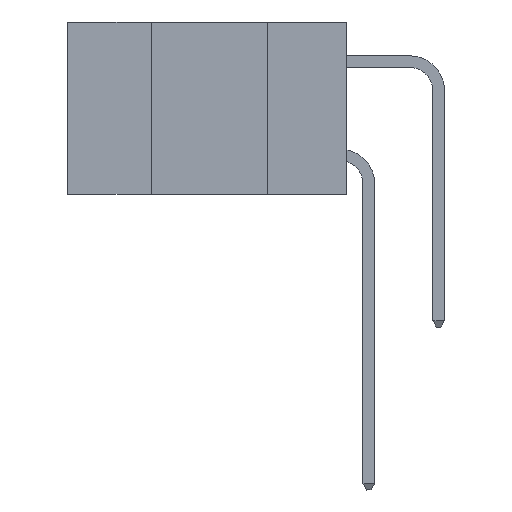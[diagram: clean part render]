
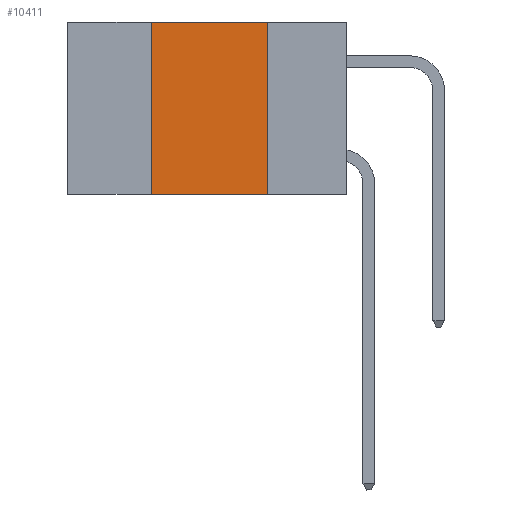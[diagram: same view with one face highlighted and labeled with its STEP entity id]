
A CAD part, left-side view. The second image highlights one B-rep face of the part: STEP entity #10411.
In plain terms, the highlighted planar face has unit normal (-1, 0, 0).
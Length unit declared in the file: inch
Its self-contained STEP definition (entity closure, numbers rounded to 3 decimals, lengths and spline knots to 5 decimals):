
#8 = ORIENTED_EDGE ( 'NONE', *, *, #389, .F. ) ;
#389 = EDGE_CURVE ( 'NONE', #8750, #6417, #7383, .T. ) ;
#1286 = EDGE_CURVE ( 'NONE', #2274, #3010, #2207, .T. ) ;
#1352 = CARTESIAN_POINT ( 'NONE',  ( 0., 0.42, 0. ) ) ;
#2051 = VECTOR ( 'NONE', #14519, 39.37008 ) ;
#2170 = CARTESIAN_POINT ( 'NONE',  ( 0., 0.42, -0.37 ) ) ;
#2207 = LINE ( 'NONE', #6857, #4844 ) ;
#2274 = VERTEX_POINT ( 'NONE', #2170 ) ;
#3010 = VERTEX_POINT ( 'NONE', #10043 ) ;
#3745 = CARTESIAN_POINT ( 'NONE',  ( 0., 0.17, 0. ) ) ;
#3824 = LINE ( 'NONE', #3745, #5643 ) ;
#4416 = DIRECTION ( 'NONE',  ( 0., -1., 0. ) ) ;
#4509 = ORIENTED_EDGE ( 'NONE', *, *, #4973, .F. ) ;
#4844 = VECTOR ( 'NONE', #4416, 39.37008 ) ;
#4973 = EDGE_CURVE ( 'NONE', #6417, #3010, #3824, .T. ) ;
#5643 = VECTOR ( 'NONE', #12863, 39.37008 ) ;
#6417 = VERTEX_POINT ( 'NONE', #11127 ) ;
#6643 = EDGE_CURVE ( 'NONE', #2274, #8750, #14911, .T. ) ;
#6857 = CARTESIAN_POINT ( 'NONE',  ( 0., 0.6, -0.37 ) ) ;
#7383 = LINE ( 'NONE', #11997, #2051 ) ;
#8090 = DIRECTION ( 'NONE',  ( 0., 0., 1. ) ) ;
#8750 = VERTEX_POINT ( 'NONE', #1352 ) ;
#8768 = ORIENTED_EDGE ( 'NONE', *, *, #1286, .T. ) ;
#9148 = CARTESIAN_POINT ( 'NONE',  ( 0., 0.42, 0. ) ) ;
#9302 = EDGE_LOOP ( 'NONE', ( #4509, #8, #12926, #8768 ) ) ;
#9333 = DIRECTION ( 'NONE',  ( 0., 0., -1. ) ) ;
#10043 = CARTESIAN_POINT ( 'NONE',  ( 0., 0.17, -0.37 ) ) ;
#10411 = ADVANCED_FACE ( 'NONE', ( #11528 ), #13747, .F. ) ;
#11127 = CARTESIAN_POINT ( 'NONE',  ( 0., 0.17, 0. ) ) ;
#11290 = VECTOR ( 'NONE', #8090, 39.37008 ) ;
#11528 = FACE_OUTER_BOUND ( 'NONE', #9302, .T. ) ;
#11997 = CARTESIAN_POINT ( 'NONE',  ( 0., 0.6, 0. ) ) ;
#12863 = DIRECTION ( 'NONE',  ( 0., 0., -1. ) ) ;
#12893 = CARTESIAN_POINT ( 'NONE',  ( 0., 0.6, 0. ) ) ;
#12926 = ORIENTED_EDGE ( 'NONE', *, *, #6643, .F. ) ;
#13747 = PLANE ( 'NONE',  #14553 ) ;
#14519 = DIRECTION ( 'NONE',  ( 0., -1., 0. ) ) ;
#14553 = AXIS2_PLACEMENT_3D ( 'NONE', #12893, #14960, #9333 ) ;
#14911 = LINE ( 'NONE', #9148, #11290 ) ;
#14960 = DIRECTION ( 'NONE',  ( 1., 0., 0. ) ) ;
